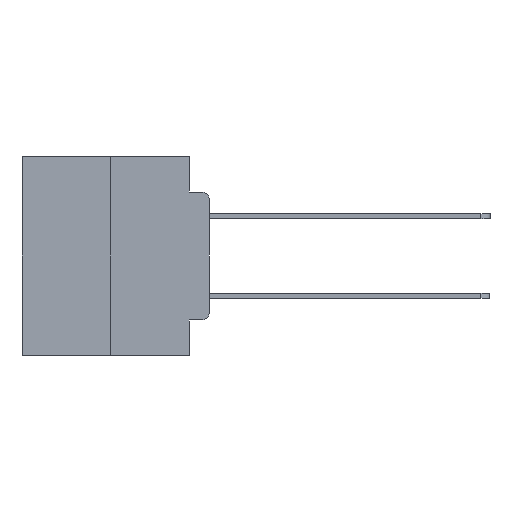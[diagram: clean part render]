
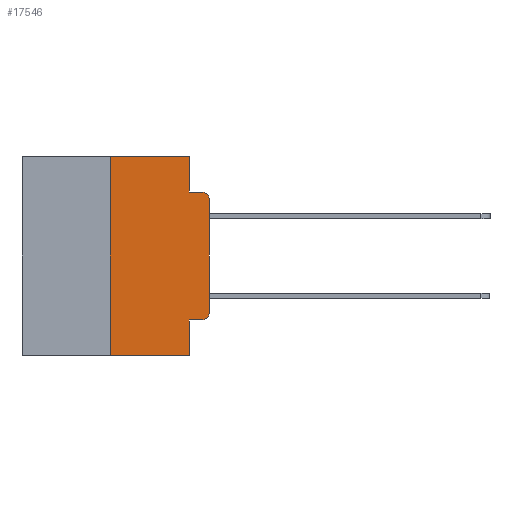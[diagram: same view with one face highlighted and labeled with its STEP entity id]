
A CAD part, left-side view. The second image highlights one B-rep face of the part: STEP entity #17546.
In plain terms, the highlighted planar face has unit normal (-1, 0, 0).
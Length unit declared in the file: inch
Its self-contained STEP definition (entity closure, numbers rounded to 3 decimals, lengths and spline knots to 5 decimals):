
#188 = CARTESIAN_POINT ( 'NONE',  ( 0., 0.02, -0.1085 ) ) ;
#452 = EDGE_CURVE ( 'NONE', #25062, #24439, #14684, .T. ) ;
#888 = CARTESIAN_POINT ( 'NONE',  ( 0., 0., -0.3915 ) ) ;
#1178 = AXIS2_PLACEMENT_3D ( 'NONE', #188, #14483, #2280 ) ;
#1665 = VERTEX_POINT ( 'NONE', #19184 ) ;
#2280 = DIRECTION ( 'NONE',  ( 0., 0., -1. ) ) ;
#2901 = CARTESIAN_POINT ( 'NONE',  ( 0., 0.25, -0.5 ) ) ;
#3167 = ORIENTED_EDGE ( 'NONE', *, *, #4437, .F. ) ;
#3360 = DIRECTION ( 'NONE',  ( 0., -1., 0. ) ) ;
#3539 = DIRECTION ( 'NONE',  ( -1., 0., 0. ) ) ;
#3815 = DIRECTION ( 'NONE',  ( 0., -1., 0. ) ) ;
#3820 = VERTEX_POINT ( 'NONE', #25347 ) ;
#3905 = CARTESIAN_POINT ( 'NONE',  ( 0., 0.051, 0. ) ) ;
#3982 = CARTESIAN_POINT ( 'NONE',  ( 0., 0.25, 0. ) ) ;
#3990 = AXIS2_PLACEMENT_3D ( 'NONE', #15694, #3539, #17753 ) ;
#4001 = VERTEX_POINT ( 'NONE', #888 ) ;
#4437 = EDGE_CURVE ( 'NONE', #24439, #18098, #24202, .T. ) ;
#4527 = AXIS2_PLACEMENT_3D ( 'NONE', #19128, #7058, #21143 ) ;
#4875 = LINE ( 'NONE', #13506, #21644 ) ;
#5476 = EDGE_CURVE ( 'NONE', #3820, #1665, #9657, .T. ) ;
#5540 = DIRECTION ( 'NONE',  ( 0., 0., 1. ) ) ;
#5553 = CARTESIAN_POINT ( 'NONE',  ( 0., 0.051, 0. ) ) ;
#5860 = CARTESIAN_POINT ( 'NONE',  ( 0., 0., -0.1085 ) ) ;
#6106 = LINE ( 'NONE', #17576, #12100 ) ;
#6825 = EDGE_CURVE ( 'NONE', #15471, #21554, #23712, .T. ) ;
#6867 = EDGE_CURVE ( 'NONE', #3820, #21554, #22459, .T. ) ;
#7058 = DIRECTION ( 'NONE',  ( 1., 0., 0. ) ) ;
#7673 = ORIENTED_EDGE ( 'NONE', *, *, #20718, .T. ) ;
#8163 = CARTESIAN_POINT ( 'NONE',  ( 0., 0.051, -0.5 ) ) ;
#8725 = CIRCLE ( 'NONE', #1178, 0.02 ) ;
#8882 = VECTOR ( 'NONE', #5540, 39.37008 ) ;
#9657 = LINE ( 'NONE', #11791, #25052 ) ;
#10493 = ORIENTED_EDGE ( 'NONE', *, *, #5476, .T. ) ;
#10671 = DIRECTION ( 'NONE',  ( 0., 0., -1. ) ) ;
#11474 = DIRECTION ( 'NONE',  ( 0., -1., 0. ) ) ;
#11628 = CARTESIAN_POINT ( 'NONE',  ( 0., 0.473, 0. ) ) ;
#11645 = CARTESIAN_POINT ( 'NONE',  ( 0., 0.051, 0. ) ) ;
#11791 = CARTESIAN_POINT ( 'NONE',  ( 0., 0.051, -0.4115 ) ) ;
#12100 = VECTOR ( 'NONE', #3360, 39.37008 ) ;
#12605 = EDGE_CURVE ( 'NONE', #18098, #13056, #6106, .T. ) ;
#13056 = VERTEX_POINT ( 'NONE', #22896 ) ;
#13506 = CARTESIAN_POINT ( 'NONE',  ( 0., 0.25, 0. ) ) ;
#13982 = ORIENTED_EDGE ( 'NONE', *, *, #24365, .F. ) ;
#14483 = DIRECTION ( 'NONE',  ( -1., 0., 0. ) ) ;
#14618 = EDGE_LOOP ( 'NONE', ( #7673, #19666, #18126, #3167, #18448, #13982, #15228, #17483, #10493, #15591 ) ) ;
#14684 = LINE ( 'NONE', #11628, #24088 ) ;
#15228 = ORIENTED_EDGE ( 'NONE', *, *, #6825, .T. ) ;
#15302 = EDGE_CURVE ( 'NONE', #22019, #13056, #8725, .T. ) ;
#15471 = VERTEX_POINT ( 'NONE', #2901 ) ;
#15528 = CIRCLE ( 'NONE', #3990, 0.02 ) ;
#15591 = ORIENTED_EDGE ( 'NONE', *, *, #26134, .T. ) ;
#15614 = CARTESIAN_POINT ( 'NONE',  ( 0., 0., 0. ) ) ;
#15694 = CARTESIAN_POINT ( 'NONE',  ( 0., 0.02, -0.3915 ) ) ;
#15982 = CARTESIAN_POINT ( 'NONE',  ( 0., 0.473, -0.5 ) ) ;
#17115 = VECTOR ( 'NONE', #26048, 39.37008 ) ;
#17483 = ORIENTED_EDGE ( 'NONE', *, *, #6867, .F. ) ;
#17546 = ADVANCED_FACE ( 'NONE', ( #23427 ), #19042, .F. ) ;
#17576 = CARTESIAN_POINT ( 'NONE',  ( 0., 0.051, -0.0885 ) ) ;
#17753 = DIRECTION ( 'NONE',  ( 0., 0., -1. ) ) ;
#18098 = VERTEX_POINT ( 'NONE', #18759 ) ;
#18126 = ORIENTED_EDGE ( 'NONE', *, *, #12605, .F. ) ;
#18387 = VECTOR ( 'NONE', #3815, 39.37008 ) ;
#18448 = ORIENTED_EDGE ( 'NONE', *, *, #452, .F. ) ;
#18759 = CARTESIAN_POINT ( 'NONE',  ( 0., 0.051, -0.0885 ) ) ;
#19042 = PLANE ( 'NONE',  #4527 ) ;
#19128 = CARTESIAN_POINT ( 'NONE',  ( 0., 0.473, 0. ) ) ;
#19184 = CARTESIAN_POINT ( 'NONE',  ( 0., 0.02, -0.4115 ) ) ;
#19646 = LINE ( 'NONE', #15614, #8882 ) ;
#19666 = ORIENTED_EDGE ( 'NONE', *, *, #15302, .T. ) ;
#20718 = EDGE_CURVE ( 'NONE', #4001, #22019, #19646, .T. ) ;
#21143 = DIRECTION ( 'NONE',  ( 0., 0., -1. ) ) ;
#21554 = VERTEX_POINT ( 'NONE', #8163 ) ;
#21644 = VECTOR ( 'NONE', #23543, 39.37008 ) ;
#22019 = VERTEX_POINT ( 'NONE', #5860 ) ;
#22459 = LINE ( 'NONE', #3905, #17115 ) ;
#22896 = CARTESIAN_POINT ( 'NONE',  ( 0., 0.02, -0.0885 ) ) ;
#23427 = FACE_OUTER_BOUND ( 'NONE', #14618, .T. ) ;
#23543 = DIRECTION ( 'NONE',  ( 0., 0., 1. ) ) ;
#23712 = LINE ( 'NONE', #15982, #18387 ) ;
#23850 = DIRECTION ( 'NONE',  ( 0., -1., 0. ) ) ;
#24088 = VECTOR ( 'NONE', #11474, 39.37008 ) ;
#24202 = LINE ( 'NONE', #5553, #24820 ) ;
#24365 = EDGE_CURVE ( 'NONE', #15471, #25062, #4875, .T. ) ;
#24439 = VERTEX_POINT ( 'NONE', #11645 ) ;
#24820 = VECTOR ( 'NONE', #10671, 39.37008 ) ;
#25052 = VECTOR ( 'NONE', #23850, 39.37008 ) ;
#25062 = VERTEX_POINT ( 'NONE', #3982 ) ;
#25347 = CARTESIAN_POINT ( 'NONE',  ( 0., 0.051, -0.4115 ) ) ;
#26048 = DIRECTION ( 'NONE',  ( 0., 0., -1. ) ) ;
#26134 = EDGE_CURVE ( 'NONE', #1665, #4001, #15528, .T. ) ;
